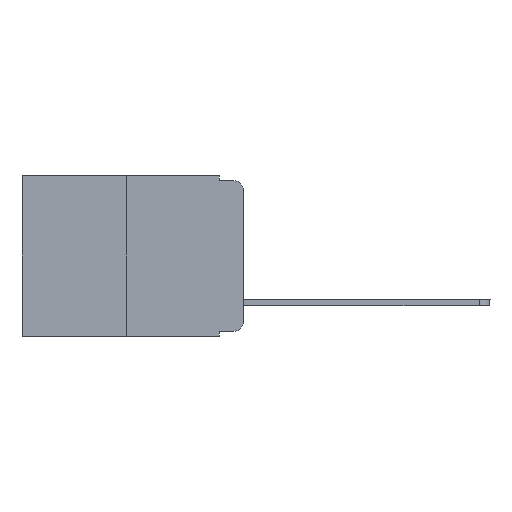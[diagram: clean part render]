
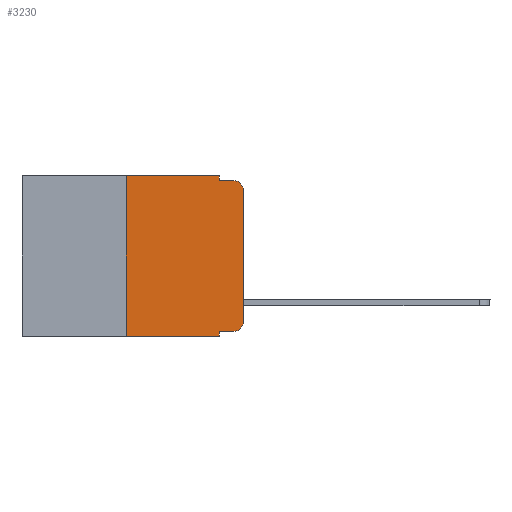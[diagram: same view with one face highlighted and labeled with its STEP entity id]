
A CAD part, left-side view. The second image highlights one B-rep face of the part: STEP entity #3230.
In plain terms, the highlighted planar face has unit normal (-1, 0, 0).
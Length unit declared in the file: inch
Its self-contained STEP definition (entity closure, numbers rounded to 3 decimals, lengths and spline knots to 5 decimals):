
#60 = CARTESIAN_POINT ( 'NONE',  ( 0., 0.051, -0.01 ) ) ;
#121 = CARTESIAN_POINT ( 'NONE',  ( 0., 0.02, -0.03 ) ) ;
#393 = DIRECTION ( 'NONE',  ( 0., -1., 0. ) ) ;
#614 = ORIENTED_EDGE ( 'NONE', *, *, #12959, .F. ) ;
#685 = VERTEX_POINT ( 'NONE', #10868 ) ;
#875 = PLANE ( 'NONE',  #13712 ) ;
#975 = VERTEX_POINT ( 'NONE', #5722 ) ;
#982 = CARTESIAN_POINT ( 'NONE',  ( 0., 0.051, 0. ) ) ;
#1043 = CIRCLE ( 'NONE', #6994, 0.02 ) ;
#1113 = EDGE_CURVE ( 'NONE', #3601, #6446, #9589, .T. ) ;
#1451 = VERTEX_POINT ( 'NONE', #1676 ) ;
#1496 = LINE ( 'NONE', #7298, #10314 ) ;
#1522 = DIRECTION ( 'NONE',  ( -1., 0., 0. ) ) ;
#1676 = CARTESIAN_POINT ( 'NONE',  ( 0., 0.25, 0. ) ) ;
#1713 = ORIENTED_EDGE ( 'NONE', *, *, #7561, .F. ) ;
#1809 = EDGE_CURVE ( 'NONE', #6024, #12564, #5693, .T. ) ;
#2101 = VECTOR ( 'NONE', #7058, 39.37008 ) ;
#2588 = CARTESIAN_POINT ( 'NONE',  ( 0., 0., 0. ) ) ;
#2679 = VERTEX_POINT ( 'NONE', #60 ) ;
#2957 = DIRECTION ( 'NONE',  ( 0., 0., -1. ) ) ;
#3093 = CARTESIAN_POINT ( 'NONE',  ( 0., 0.25, 0. ) ) ;
#3230 = ADVANCED_FACE ( 'NONE', ( #11072 ), #875, .F. ) ;
#3417 = EDGE_CURVE ( 'NONE', #1451, #9771, #6076, .T. ) ;
#3508 = CARTESIAN_POINT ( 'NONE',  ( 0., 0.25, -0.343 ) ) ;
#3577 = CARTESIAN_POINT ( 'NONE',  ( 0., 0.051, -0.01 ) ) ;
#3601 = VERTEX_POINT ( 'NONE', #14400 ) ;
#3991 = CARTESIAN_POINT ( 'NONE',  ( 0., 0.473, 0. ) ) ;
#4053 = LINE ( 'NONE', #3093, #5544 ) ;
#4209 = VECTOR ( 'NONE', #8007, 39.37008 ) ;
#4341 = LINE ( 'NONE', #5309, #4738 ) ;
#4420 = VERTEX_POINT ( 'NONE', #3508 ) ;
#4724 = DIRECTION ( 'NONE',  ( 0., -1., 0. ) ) ;
#4738 = VECTOR ( 'NONE', #12316, 39.37008 ) ;
#4987 = DIRECTION ( 'NONE',  ( 0., 0., -1. ) ) ;
#5309 = CARTESIAN_POINT ( 'NONE',  ( 0., 0.051, 0. ) ) ;
#5349 = ORIENTED_EDGE ( 'NONE', *, *, #1809, .T. ) ;
#5541 = CARTESIAN_POINT ( 'NONE',  ( 0., 0.051, -0.333 ) ) ;
#5544 = VECTOR ( 'NONE', #12103, 39.37008 ) ;
#5693 = LINE ( 'NONE', #5541, #4209 ) ;
#5722 = CARTESIAN_POINT ( 'NONE',  ( 0., 0.051, -0.343 ) ) ;
#5928 = CARTESIAN_POINT ( 'NONE',  ( 0., 0.02, -0.333 ) ) ;
#6024 = VERTEX_POINT ( 'NONE', #13760 ) ;
#6076 = LINE ( 'NONE', #11511, #8950 ) ;
#6446 = VERTEX_POINT ( 'NONE', #7036 ) ;
#6909 = CARTESIAN_POINT ( 'NONE',  ( 0., 0.051, 0. ) ) ;
#6952 = DIRECTION ( 'NONE',  ( 0., 0., -1. ) ) ;
#6994 = AXIS2_PLACEMENT_3D ( 'NONE', #121, #1522, #6952 ) ;
#7036 = CARTESIAN_POINT ( 'NONE',  ( 0., 0., -0.03 ) ) ;
#7058 = DIRECTION ( 'NONE',  ( 0., 0., -1. ) ) ;
#7135 = DIRECTION ( 'NONE',  ( 0., 0., 1. ) ) ;
#7223 = VECTOR ( 'NONE', #7905, 39.37008 ) ;
#7298 = CARTESIAN_POINT ( 'NONE',  ( 0., 0.473, -0.343 ) ) ;
#7471 = ORIENTED_EDGE ( 'NONE', *, *, #8173, .F. ) ;
#7561 = EDGE_CURVE ( 'NONE', #9771, #2679, #10550, .T. ) ;
#7905 = DIRECTION ( 'NONE',  ( 0., -1., 0. ) ) ;
#8007 = DIRECTION ( 'NONE',  ( 0., -1., 0. ) ) ;
#8173 = EDGE_CURVE ( 'NONE', #6024, #975, #4341, .T. ) ;
#8950 = VECTOR ( 'NONE', #4724, 39.37008 ) ;
#8996 = VECTOR ( 'NONE', #7135, 39.37008 ) ;
#9102 = LINE ( 'NONE', #3577, #7223 ) ;
#9536 = CARTESIAN_POINT ( 'NONE',  ( 0., 0.02, -0.313 ) ) ;
#9589 = LINE ( 'NONE', #2588, #8996 ) ;
#9771 = VERTEX_POINT ( 'NONE', #982 ) ;
#10220 = EDGE_LOOP ( 'NONE', ( #11847, #13089, #614, #1713, #14425, #10456, #11044, #7471, #5349, #14087 ) ) ;
#10314 = VECTOR ( 'NONE', #393, 39.37008 ) ;
#10456 = ORIENTED_EDGE ( 'NONE', *, *, #14043, .F. ) ;
#10550 = LINE ( 'NONE', #6909, #2101 ) ;
#10551 = AXIS2_PLACEMENT_3D ( 'NONE', #9536, #13925, #4987 ) ;
#10868 = CARTESIAN_POINT ( 'NONE',  ( 0., 0.02, -0.01 ) ) ;
#11044 = ORIENTED_EDGE ( 'NONE', *, *, #13019, .T. ) ;
#11072 = FACE_OUTER_BOUND ( 'NONE', #10220, .T. ) ;
#11511 = CARTESIAN_POINT ( 'NONE',  ( 0., 0.473, 0. ) ) ;
#11762 = EDGE_CURVE ( 'NONE', #12564, #3601, #13877, .T. ) ;
#11847 = ORIENTED_EDGE ( 'NONE', *, *, #1113, .T. ) ;
#12103 = DIRECTION ( 'NONE',  ( 0., 0., 1. ) ) ;
#12316 = DIRECTION ( 'NONE',  ( 0., 0., -1. ) ) ;
#12564 = VERTEX_POINT ( 'NONE', #5928 ) ;
#12959 = EDGE_CURVE ( 'NONE', #2679, #685, #9102, .T. ) ;
#13019 = EDGE_CURVE ( 'NONE', #4420, #975, #1496, .T. ) ;
#13089 = ORIENTED_EDGE ( 'NONE', *, *, #14323, .T. ) ;
#13153 = DIRECTION ( 'NONE',  ( 1., 0., 0. ) ) ;
#13712 = AXIS2_PLACEMENT_3D ( 'NONE', #3991, #13153, #2957 ) ;
#13760 = CARTESIAN_POINT ( 'NONE',  ( 0., 0.051, -0.333 ) ) ;
#13877 = CIRCLE ( 'NONE', #10551, 0.02 ) ;
#13925 = DIRECTION ( 'NONE',  ( -1., 0., 0. ) ) ;
#14043 = EDGE_CURVE ( 'NONE', #4420, #1451, #4053, .T. ) ;
#14087 = ORIENTED_EDGE ( 'NONE', *, *, #11762, .T. ) ;
#14323 = EDGE_CURVE ( 'NONE', #6446, #685, #1043, .T. ) ;
#14400 = CARTESIAN_POINT ( 'NONE',  ( 0., 0., -0.313 ) ) ;
#14425 = ORIENTED_EDGE ( 'NONE', *, *, #3417, .F. ) ;
